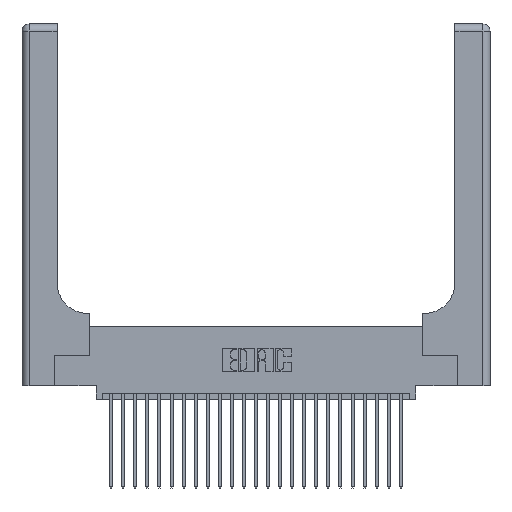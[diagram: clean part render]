
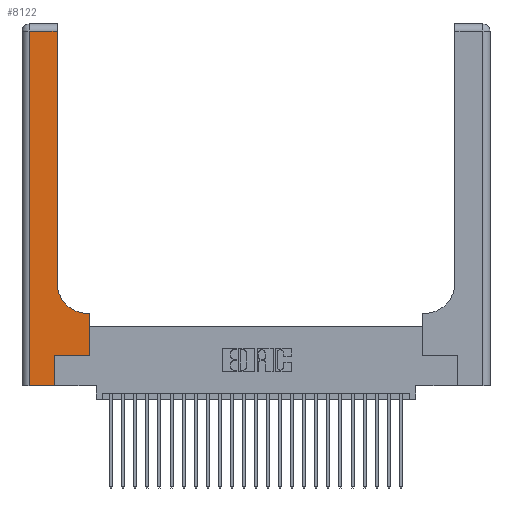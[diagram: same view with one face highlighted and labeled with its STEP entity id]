
A CAD part, top view. The second image highlights one B-rep face of the part: STEP entity #8122.
In plain terms, the highlighted planar face has unit normal (0, 0, 1).
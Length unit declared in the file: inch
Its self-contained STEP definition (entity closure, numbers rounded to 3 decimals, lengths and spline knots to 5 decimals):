
#681 = ORIENTED_EDGE ( 'NONE', *, *, #11363, .T. ) ;
#743 = CARTESIAN_POINT ( 'NONE',  ( 0.06, 2.94, 0.37 ) ) ;
#1505 = CARTESIAN_POINT ( 'NONE',  ( 0.2915, 3., 0.37 ) ) ;
#2255 = VERTEX_POINT ( 'NONE', #12059 ) ;
#2430 = VERTEX_POINT ( 'NONE', #3521 ) ;
#2528 = EDGE_CURVE ( 'NONE', #22830, #3480, #18381, .T. ) ;
#2662 = VECTOR ( 'NONE', #16771, 39.37008 ) ;
#3480 = VERTEX_POINT ( 'NONE', #20418 ) ;
#3521 = CARTESIAN_POINT ( 'NONE',  ( 0.5415, 0.6, 0.37 ) ) ;
#3527 = LINE ( 'NONE', #1505, #25237 ) ;
#4600 = EDGE_CURVE ( 'NONE', #2430, #16143, #20958, .T. ) ;
#4626 = PLANE ( 'NONE',  #14943 ) ;
#4972 = EDGE_CURVE ( 'NONE', #8407, #6482, #18942, .T. ) ;
#5712 = LINE ( 'NONE', #17847, #17819 ) ;
#6482 = VERTEX_POINT ( 'NONE', #15788 ) ;
#7384 = EDGE_CURVE ( 'NONE', #6482, #2255, #5712, .T. ) ;
#7674 = DIRECTION ( 'NONE',  ( 1., 0., 0. ) ) ;
#7778 = CARTESIAN_POINT ( 'NONE',  ( 0.5415, 0.85, 0.37 ) ) ;
#7893 = LINE ( 'NONE', #12319, #9498 ) ;
#7945 = VECTOR ( 'NONE', #9064, 39.37008 ) ;
#8022 = DIRECTION ( 'NONE',  ( 0., 1., 0. ) ) ;
#8122 = ADVANCED_FACE ( 'NONE', ( #19938 ), #4626, .F. ) ;
#8407 = VERTEX_POINT ( 'NONE', #8693 ) ;
#8581 = LINE ( 'NONE', #12961, #2662 ) ;
#8592 = EDGE_CURVE ( 'NONE', #15372, #22830, #8581, .T. ) ;
#8693 = CARTESIAN_POINT ( 'NONE',  ( 0.269, 0.25, 0.37 ) ) ;
#9064 = DIRECTION ( 'NONE',  ( -1., 0., 0. ) ) ;
#9483 = ORIENTED_EDGE ( 'NONE', *, *, #7384, .T. ) ;
#9498 = VECTOR ( 'NONE', #25124, 39.37008 ) ;
#9772 = EDGE_LOOP ( 'NONE', ( #681, #14847, #11384, #10145, #21090, #26609, #9483, #20477, #21167 ) ) ;
#10070 = VECTOR ( 'NONE', #25199, 39.37008 ) ;
#10145 = ORIENTED_EDGE ( 'NONE', *, *, #2528, .T. ) ;
#11363 = EDGE_CURVE ( 'NONE', #16143, #26681, #3527, .T. ) ;
#11384 = ORIENTED_EDGE ( 'NONE', *, *, #8592, .T. ) ;
#11456 = EDGE_CURVE ( 'NONE', #2255, #2430, #27198, .T. ) ;
#12059 = CARTESIAN_POINT ( 'NONE',  ( 0.5585, 0.6, 0.37 ) ) ;
#12179 = CARTESIAN_POINT ( 'NONE',  ( 0.2915, 0.85, 0.37 ) ) ;
#12319 = CARTESIAN_POINT ( 'NONE',  ( 0.269, 0., 0.37 ) ) ;
#12961 = CARTESIAN_POINT ( 'NONE',  ( 0.06, 3., 0.37 ) ) ;
#14126 = CARTESIAN_POINT ( 'NONE',  ( 0., 0., 0.37 ) ) ;
#14847 = ORIENTED_EDGE ( 'NONE', *, *, #24965, .T. ) ;
#14943 = AXIS2_PLACEMENT_3D ( 'NONE', #23658, #23764, #21627 ) ;
#15093 = CARTESIAN_POINT ( 'NONE',  ( 0.2915, 2.94, 0.37 ) ) ;
#15372 = VERTEX_POINT ( 'NONE', #743 ) ;
#15788 = CARTESIAN_POINT ( 'NONE',  ( 0.5585, 0.25, 0.37 ) ) ;
#16127 = DIRECTION ( 'NONE',  ( 1., 0., 0. ) ) ;
#16143 = VERTEX_POINT ( 'NONE', #12179 ) ;
#16583 = CARTESIAN_POINT ( 'NONE',  ( 0.2915, 0.6, 0.37 ) ) ;
#16771 = DIRECTION ( 'NONE',  ( 0., -1., 0. ) ) ;
#17819 = VECTOR ( 'NONE', #18225, 39.37008 ) ;
#17847 = CARTESIAN_POINT ( 'NONE',  ( 0.5585, 0.25, 0.37 ) ) ;
#18225 = DIRECTION ( 'NONE',  ( 0., 1., 0. ) ) ;
#18381 = LINE ( 'NONE', #14126, #20678 ) ;
#18942 = LINE ( 'NONE', #21900, #26568 ) ;
#19938 = FACE_OUTER_BOUND ( 'NONE', #9772, .T. ) ;
#20418 = CARTESIAN_POINT ( 'NONE',  ( 0.269, 0., 0.37 ) ) ;
#20477 = ORIENTED_EDGE ( 'NONE', *, *, #11456, .T. ) ;
#20678 = VECTOR ( 'NONE', #16127, 39.37008 ) ;
#20702 = AXIS2_PLACEMENT_3D ( 'NONE', #7778, #22568, #7674 ) ;
#20958 = CIRCLE ( 'NONE', #20702, 0.25 ) ;
#21090 = ORIENTED_EDGE ( 'NONE', *, *, #26013, .T. ) ;
#21167 = ORIENTED_EDGE ( 'NONE', *, *, #4600, .T. ) ;
#21627 = DIRECTION ( 'NONE',  ( -1., 0., 0. ) ) ;
#21900 = CARTESIAN_POINT ( 'NONE',  ( 0.269, 0.25, 0.37 ) ) ;
#22568 = DIRECTION ( 'NONE',  ( 0., 0., -1. ) ) ;
#22830 = VERTEX_POINT ( 'NONE', #26174 ) ;
#23658 = CARTESIAN_POINT ( 'NONE',  ( 0., 3., 0.37 ) ) ;
#23729 = LINE ( 'NONE', #25546, #7945 ) ;
#23764 = DIRECTION ( 'NONE',  ( 0., 0., -1. ) ) ;
#24965 = EDGE_CURVE ( 'NONE', #26681, #15372, #23729, .T. ) ;
#25124 = DIRECTION ( 'NONE',  ( 0., 1., 0. ) ) ;
#25199 = DIRECTION ( 'NONE',  ( -1., 0., 0. ) ) ;
#25237 = VECTOR ( 'NONE', #8022, 39.37008 ) ;
#25546 = CARTESIAN_POINT ( 'NONE',  ( 0., 2.94, 0.37 ) ) ;
#26013 = EDGE_CURVE ( 'NONE', #3480, #8407, #7893, .T. ) ;
#26174 = CARTESIAN_POINT ( 'NONE',  ( 0.06, 0., 0.37 ) ) ;
#26438 = DIRECTION ( 'NONE',  ( 1., 0., 0. ) ) ;
#26568 = VECTOR ( 'NONE', #26438, 39.37008 ) ;
#26609 = ORIENTED_EDGE ( 'NONE', *, *, #4972, .T. ) ;
#26681 = VERTEX_POINT ( 'NONE', #15093 ) ;
#27198 = LINE ( 'NONE', #16583, #10070 ) ;
